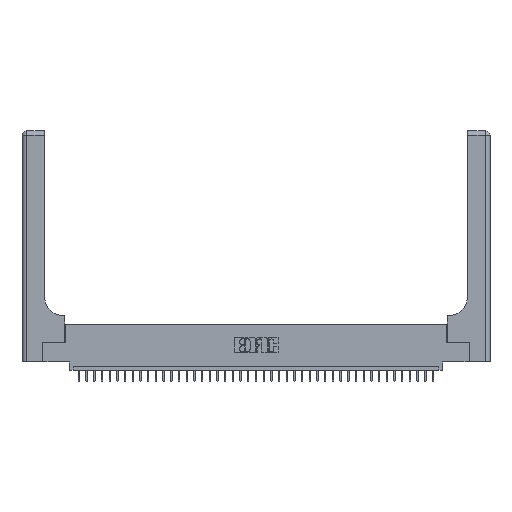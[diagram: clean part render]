
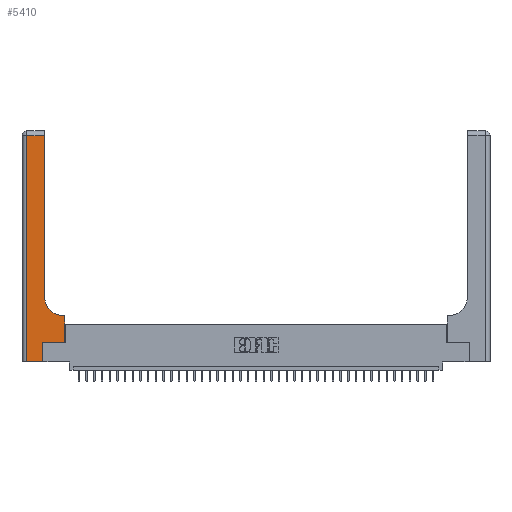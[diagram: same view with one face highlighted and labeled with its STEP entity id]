
A CAD part, top view. The second image highlights one B-rep face of the part: STEP entity #5410.
In plain terms, the highlighted planar face has unit normal (0, 0, 1).
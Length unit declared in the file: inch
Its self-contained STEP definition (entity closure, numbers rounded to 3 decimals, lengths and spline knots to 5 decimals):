
#123 = CARTESIAN_POINT ( 'NONE',  ( 0., 2.94, 0.37 ) ) ;
#682 = CARTESIAN_POINT ( 'NONE',  ( 0.269, 0., 0.37 ) ) ;
#1881 = ORIENTED_EDGE ( 'NONE', *, *, #18486, .T. ) ;
#2394 = DIRECTION ( 'NONE',  ( 0., -1., 0. ) ) ;
#2514 = EDGE_CURVE ( 'NONE', #30262, #23477, #13716, .T. ) ;
#4020 = EDGE_CURVE ( 'NONE', #10552, #29844, #11030, .T. ) ;
#4274 = DIRECTION ( 'NONE',  ( 1., 0., 0. ) ) ;
#5260 = VECTOR ( 'NONE', #32371, 39.37008 ) ;
#5410 = ADVANCED_FACE ( 'NONE', ( #8171 ), #38609, .F. ) ;
#5552 = EDGE_CURVE ( 'NONE', #23477, #12170, #8766, .T. ) ;
#6897 = ORIENTED_EDGE ( 'NONE', *, *, #39568, .T. ) ;
#7309 = CARTESIAN_POINT ( 'NONE',  ( 0., 0., 0.37 ) ) ;
#7359 = CARTESIAN_POINT ( 'NONE',  ( 0., 3., 0.37 ) ) ;
#8171 = FACE_OUTER_BOUND ( 'NONE', #39091, .T. ) ;
#8336 = LINE ( 'NONE', #28129, #26202 ) ;
#8766 = LINE ( 'NONE', #11810, #39120 ) ;
#8962 = ORIENTED_EDGE ( 'NONE', *, *, #2514, .T. ) ;
#9067 = CARTESIAN_POINT ( 'NONE',  ( 0.5585, 0.25, 0.37 ) ) ;
#9808 = VECTOR ( 'NONE', #4274, 39.37008 ) ;
#9910 = CARTESIAN_POINT ( 'NONE',  ( 0.06, 2.94, 0.37 ) ) ;
#10047 = VERTEX_POINT ( 'NONE', #39475 ) ;
#10552 = VERTEX_POINT ( 'NONE', #37134 ) ;
#10634 = ORIENTED_EDGE ( 'NONE', *, *, #14445, .T. ) ;
#10841 = DIRECTION ( 'NONE',  ( 0., 1., 0. ) ) ;
#11030 = LINE ( 'NONE', #25833, #29300 ) ;
#11810 = CARTESIAN_POINT ( 'NONE',  ( 0.2915, 0.6, 0.37 ) ) ;
#12170 = VERTEX_POINT ( 'NONE', #38793 ) ;
#13061 = DIRECTION ( 'NONE',  ( 0., 1., 0. ) ) ;
#13610 = DIRECTION ( 'NONE',  ( 0., 0., -1. ) ) ;
#13716 = LINE ( 'NONE', #35211, #5260 ) ;
#13833 = ORIENTED_EDGE ( 'NONE', *, *, #5552, .T. ) ;
#14445 = EDGE_CURVE ( 'NONE', #10047, #35852, #19087, .T. ) ;
#15051 = DIRECTION ( 'NONE',  ( -1., 0., 0. ) ) ;
#17178 = VECTOR ( 'NONE', #2394, 39.37008 ) ;
#17946 = EDGE_CURVE ( 'NONE', #12170, #10552, #26813, .T. ) ;
#18486 = EDGE_CURVE ( 'NONE', #27275, #10047, #23893, .T. ) ;
#18517 = ORIENTED_EDGE ( 'NONE', *, *, #17946, .T. ) ;
#18702 = VERTEX_POINT ( 'NONE', #31170 ) ;
#19087 = LINE ( 'NONE', #7309, #9808 ) ;
#19946 = EDGE_CURVE ( 'NONE', #18702, #30262, #8336, .T. ) ;
#20387 = EDGE_CURVE ( 'NONE', #35852, #18702, #28478, .T. ) ;
#22997 = VECTOR ( 'NONE', #13061, 39.37008 ) ;
#23477 = VERTEX_POINT ( 'NONE', #36347 ) ;
#23893 = LINE ( 'NONE', #32820, #17178 ) ;
#24709 = CARTESIAN_POINT ( 'NONE',  ( 0.2915, 2.94, 0.37 ) ) ;
#24883 = DIRECTION ( 'NONE',  ( 1., 0., 0. ) ) ;
#25833 = CARTESIAN_POINT ( 'NONE',  ( 0.2915, 3., 0.37 ) ) ;
#26202 = VECTOR ( 'NONE', #24883, 39.37008 ) ;
#26603 = DIRECTION ( 'NONE',  ( 0., 0., -1. ) ) ;
#26813 = CIRCLE ( 'NONE', #30058, 0.25 ) ;
#27076 = VECTOR ( 'NONE', #37660, 39.37008 ) ;
#27275 = VERTEX_POINT ( 'NONE', #9910 ) ;
#28129 = CARTESIAN_POINT ( 'NONE',  ( 0.269, 0.25, 0.37 ) ) ;
#28478 = LINE ( 'NONE', #682, #22997 ) ;
#28726 = ORIENTED_EDGE ( 'NONE', *, *, #20387, .T. ) ;
#29057 = DIRECTION ( 'NONE',  ( -1., 0., 0. ) ) ;
#29300 = VECTOR ( 'NONE', #10841, 39.37008 ) ;
#29364 = AXIS2_PLACEMENT_3D ( 'NONE', #7359, #26603, #29057 ) ;
#29418 = DIRECTION ( 'NONE',  ( 1., 0., 0. ) ) ;
#29844 = VERTEX_POINT ( 'NONE', #24709 ) ;
#30058 = AXIS2_PLACEMENT_3D ( 'NONE', #32263, #13610, #29418 ) ;
#30262 = VERTEX_POINT ( 'NONE', #9067 ) ;
#31170 = CARTESIAN_POINT ( 'NONE',  ( 0.269, 0.25, 0.37 ) ) ;
#32263 = CARTESIAN_POINT ( 'NONE',  ( 0.5415, 0.85, 0.37 ) ) ;
#32371 = DIRECTION ( 'NONE',  ( 0., 1., 0. ) ) ;
#32820 = CARTESIAN_POINT ( 'NONE',  ( 0.06, 3., 0.37 ) ) ;
#32879 = CARTESIAN_POINT ( 'NONE',  ( 0.269, 0., 0.37 ) ) ;
#35211 = CARTESIAN_POINT ( 'NONE',  ( 0.5585, 0.25, 0.37 ) ) ;
#35852 = VERTEX_POINT ( 'NONE', #32879 ) ;
#36297 = ORIENTED_EDGE ( 'NONE', *, *, #4020, .T. ) ;
#36347 = CARTESIAN_POINT ( 'NONE',  ( 0.5585, 0.6, 0.37 ) ) ;
#36685 = ORIENTED_EDGE ( 'NONE', *, *, #19946, .T. ) ;
#37134 = CARTESIAN_POINT ( 'NONE',  ( 0.2915, 0.85, 0.37 ) ) ;
#37660 = DIRECTION ( 'NONE',  ( -1., 0., 0. ) ) ;
#38609 = PLANE ( 'NONE',  #29364 ) ;
#38793 = CARTESIAN_POINT ( 'NONE',  ( 0.5415, 0.6, 0.37 ) ) ;
#39091 = EDGE_LOOP ( 'NONE', ( #36297, #6897, #1881, #10634, #28726, #36685, #8962, #13833, #18517 ) ) ;
#39120 = VECTOR ( 'NONE', #15051, 39.37008 ) ;
#39475 = CARTESIAN_POINT ( 'NONE',  ( 0.06, 0., 0.37 ) ) ;
#39568 = EDGE_CURVE ( 'NONE', #29844, #27275, #40092, .T. ) ;
#40092 = LINE ( 'NONE', #123, #27076 ) ;
